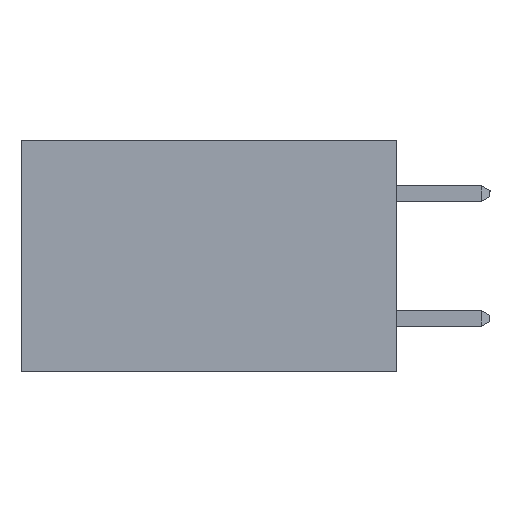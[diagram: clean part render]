
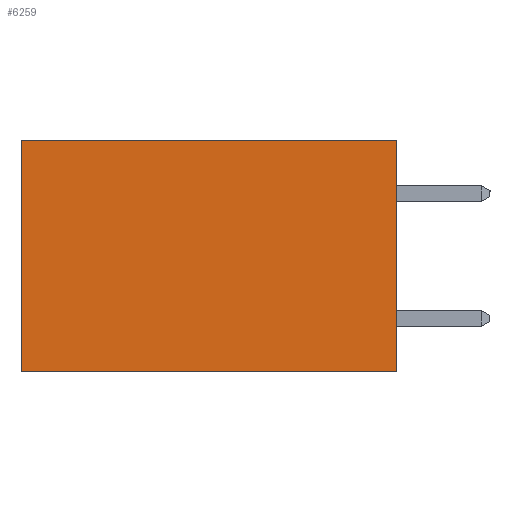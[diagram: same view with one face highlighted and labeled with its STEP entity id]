
A CAD part, left-side view. The second image highlights one B-rep face of the part: STEP entity #6259.
In plain terms, the highlighted planar face has unit normal (-1, 0, 0).
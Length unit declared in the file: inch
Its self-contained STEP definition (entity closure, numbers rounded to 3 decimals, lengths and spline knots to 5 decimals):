
#295 = FACE_OUTER_BOUND ( 'NONE', #5424, .T. ) ;
#513 = CARTESIAN_POINT ( 'NONE',  ( 0.2615, 0., 0. ) ) ;
#923 = CARTESIAN_POINT ( 'NONE',  ( 0.2615, 0., -0.37 ) ) ;
#2439 = VECTOR ( 'NONE', #3473, 39.37008 ) ;
#2631 = DIRECTION ( 'NONE',  ( 1., 0., 0. ) ) ;
#2683 = PLANE ( 'NONE',  #3603 ) ;
#2722 = CARTESIAN_POINT ( 'NONE',  ( 0.2615, 0., -0.37 ) ) ;
#2802 = EDGE_CURVE ( 'NONE', #5552, #8767, #6216, .T. ) ;
#2965 = CARTESIAN_POINT ( 'NONE',  ( 0.2615, 0., -0.37 ) ) ;
#2974 = ORIENTED_EDGE ( 'NONE', *, *, #2802, .T. ) ;
#3471 = CARTESIAN_POINT ( 'NONE',  ( 0.2615, 0., 0. ) ) ;
#3473 = DIRECTION ( 'NONE',  ( 0., 1., 0. ) ) ;
#3603 = AXIS2_PLACEMENT_3D ( 'NONE', #5888, #2631, #9011 ) ;
#3845 = EDGE_CURVE ( 'NONE', #5552, #9761, #5986, .T. ) ;
#4218 = CARTESIAN_POINT ( 'NONE',  ( 0.2615, 0.6, 0. ) ) ;
#4771 = CARTESIAN_POINT ( 'NONE',  ( 0.2615, 0.6, -0.37 ) ) ;
#4866 = LINE ( 'NONE', #4771, #5638 ) ;
#5424 = EDGE_LOOP ( 'NONE', ( #9260, #8085, #8047, #2974 ) ) ;
#5552 = VERTEX_POINT ( 'NONE', #3471 ) ;
#5638 = VECTOR ( 'NONE', #7263, 39.37008 ) ;
#5888 = CARTESIAN_POINT ( 'NONE',  ( 0.2615, 0., -0.37 ) ) ;
#5986 = LINE ( 'NONE', #2965, #8233 ) ;
#6216 = LINE ( 'NONE', #513, #9255 ) ;
#6246 = EDGE_CURVE ( 'NONE', #9761, #8327, #8149, .T. ) ;
#6259 = ADVANCED_FACE ( 'NONE', ( #295 ), #2683, .F. ) ;
#7263 = DIRECTION ( 'NONE',  ( 0., 0., -1. ) ) ;
#8047 = ORIENTED_EDGE ( 'NONE', *, *, #3845, .F. ) ;
#8085 = ORIENTED_EDGE ( 'NONE', *, *, #6246, .F. ) ;
#8149 = LINE ( 'NONE', #2722, #2439 ) ;
#8233 = VECTOR ( 'NONE', #9297, 39.37008 ) ;
#8327 = VERTEX_POINT ( 'NONE', #10297 ) ;
#8767 = VERTEX_POINT ( 'NONE', #4218 ) ;
#9011 = DIRECTION ( 'NONE',  ( 0., 0., -1. ) ) ;
#9255 = VECTOR ( 'NONE', #9424, 39.37008 ) ;
#9260 = ORIENTED_EDGE ( 'NONE', *, *, #9556, .T. ) ;
#9297 = DIRECTION ( 'NONE',  ( 0., 0., -1. ) ) ;
#9424 = DIRECTION ( 'NONE',  ( 0., 1., 0. ) ) ;
#9556 = EDGE_CURVE ( 'NONE', #8767, #8327, #4866, .T. ) ;
#9761 = VERTEX_POINT ( 'NONE', #923 ) ;
#10297 = CARTESIAN_POINT ( 'NONE',  ( 0.2615, 0.6, -0.37 ) ) ;
